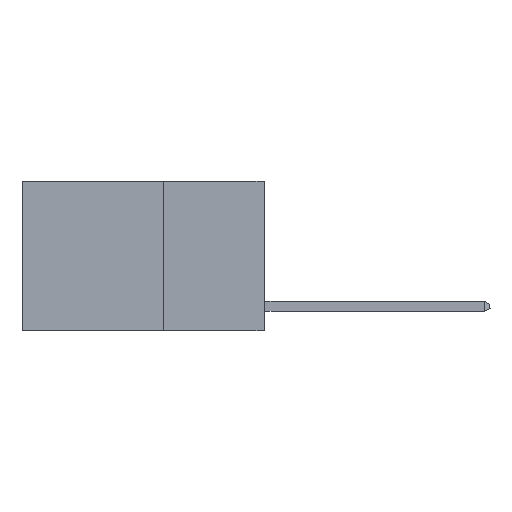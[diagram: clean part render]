
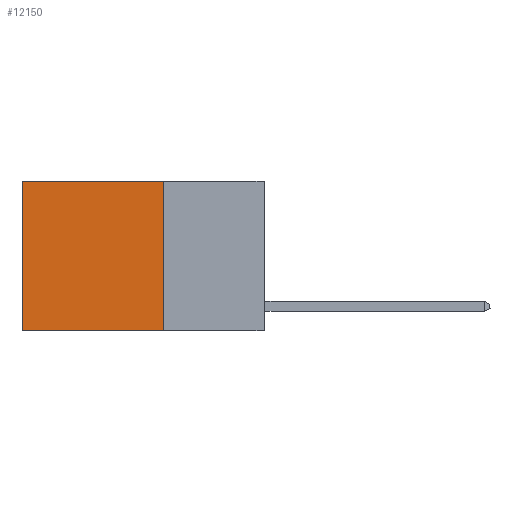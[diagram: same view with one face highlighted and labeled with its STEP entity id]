
A CAD part, left-side view. The second image highlights one B-rep face of the part: STEP entity #12150.
In plain terms, the highlighted planar face has unit normal (-1, 0, 0).
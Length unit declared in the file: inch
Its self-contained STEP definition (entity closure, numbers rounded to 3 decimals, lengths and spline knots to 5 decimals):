
#627 = LINE ( 'NONE', #15212, #17390 ) ;
#1229 = CARTESIAN_POINT ( 'NONE',  ( 0.2625, 0.25, 0. ) ) ;
#1487 = LINE ( 'NONE', #15417, #22403 ) ;
#2010 = AXIS2_PLACEMENT_3D ( 'NONE', #2849, #16425, #10289 ) ;
#2249 = CARTESIAN_POINT ( 'NONE',  ( 0.2625, 0.25, -0.37 ) ) ;
#2849 = CARTESIAN_POINT ( 'NONE',  ( 0.2625, 0.25, 0. ) ) ;
#4476 = LINE ( 'NONE', #15389, #7246 ) ;
#5002 = EDGE_CURVE ( 'NONE', #11220, #10244, #627, .T. ) ;
#5142 = ORIENTED_EDGE ( 'NONE', *, *, #18538, .T. ) ;
#7246 = VECTOR ( 'NONE', #11888, 39.37008 ) ;
#7871 = FACE_OUTER_BOUND ( 'NONE', #23861, .T. ) ;
#10244 = VERTEX_POINT ( 'NONE', #21056 ) ;
#10289 = DIRECTION ( 'NONE',  ( 0., 0., -1. ) ) ;
#11098 = VERTEX_POINT ( 'NONE', #16006 ) ;
#11220 = VERTEX_POINT ( 'NONE', #11416 ) ;
#11416 = CARTESIAN_POINT ( 'NONE',  ( 0.2625, 0.25, 0. ) ) ;
#11888 = DIRECTION ( 'NONE',  ( 0., 0., -1. ) ) ;
#12150 = ADVANCED_FACE ( 'NONE', ( #7871 ), #15239, .F. ) ;
#12679 = VERTEX_POINT ( 'NONE', #2249 ) ;
#13615 = DIRECTION ( 'NONE',  ( 0., 1., 0. ) ) ;
#15030 = EDGE_CURVE ( 'NONE', #11220, #12679, #17943, .T. ) ;
#15212 = CARTESIAN_POINT ( 'NONE',  ( 0.2625, 0.25, 0. ) ) ;
#15239 = PLANE ( 'NONE',  #2010 ) ;
#15319 = VECTOR ( 'NONE', #18325, 39.37008 ) ;
#15389 = CARTESIAN_POINT ( 'NONE',  ( 0.2625, 0.6, 0. ) ) ;
#15417 = CARTESIAN_POINT ( 'NONE',  ( 0.2625, 0.25, -0.37 ) ) ;
#16006 = CARTESIAN_POINT ( 'NONE',  ( 0.2625, 0.6, -0.37 ) ) ;
#16202 = EDGE_CURVE ( 'NONE', #12679, #11098, #1487, .T. ) ;
#16425 = DIRECTION ( 'NONE',  ( 1., 0., 0. ) ) ;
#17390 = VECTOR ( 'NONE', #18944, 39.37008 ) ;
#17943 = LINE ( 'NONE', #1229, #15319 ) ;
#18325 = DIRECTION ( 'NONE',  ( 0., 0., -1. ) ) ;
#18447 = ORIENTED_EDGE ( 'NONE', *, *, #5002, .T. ) ;
#18538 = EDGE_CURVE ( 'NONE', #10244, #11098, #4476, .T. ) ;
#18944 = DIRECTION ( 'NONE',  ( 0., 1., 0. ) ) ;
#19061 = ORIENTED_EDGE ( 'NONE', *, *, #16202, .F. ) ;
#20929 = ORIENTED_EDGE ( 'NONE', *, *, #15030, .F. ) ;
#21056 = CARTESIAN_POINT ( 'NONE',  ( 0.2625, 0.6, 0. ) ) ;
#22403 = VECTOR ( 'NONE', #13615, 39.37008 ) ;
#23861 = EDGE_LOOP ( 'NONE', ( #5142, #19061, #20929, #18447 ) ) ;
